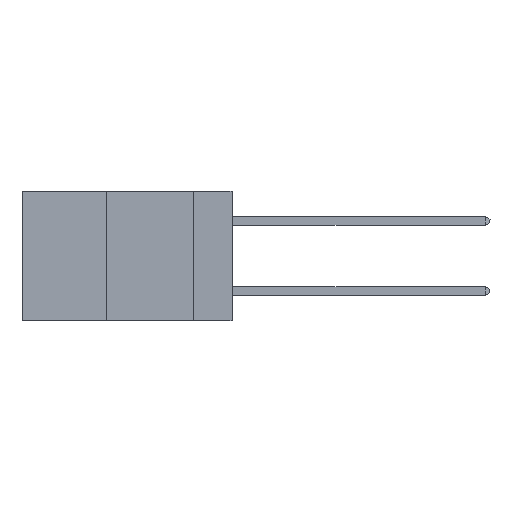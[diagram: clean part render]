
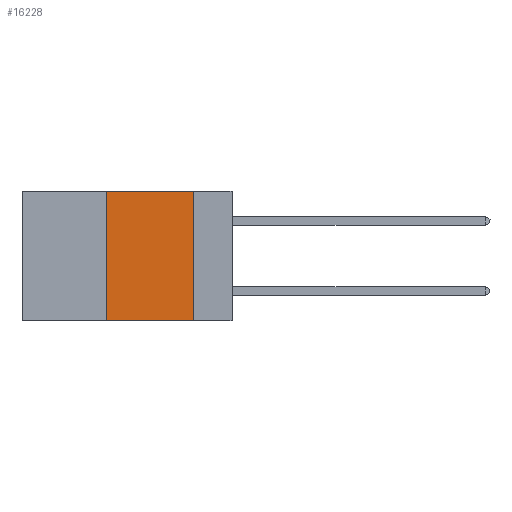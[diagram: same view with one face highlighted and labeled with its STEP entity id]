
A CAD part, left-side view. The second image highlights one B-rep face of the part: STEP entity #16228.
In plain terms, the highlighted planar face has unit normal (-1, 0, 0).
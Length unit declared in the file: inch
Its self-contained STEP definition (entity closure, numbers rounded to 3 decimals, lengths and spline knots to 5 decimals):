
#577 = EDGE_CURVE ( 'NONE', #12885, #24076, #1786, .T. ) ;
#1786 = LINE ( 'NONE', #29263, #32819 ) ;
#3264 = VECTOR ( 'NONE', #8563, 39.37008 ) ;
#3924 = CARTESIAN_POINT ( 'NONE',  ( 0., 0.36, -0.37 ) ) ;
#4252 = CARTESIAN_POINT ( 'NONE',  ( 0., 0.11, -0.37 ) ) ;
#4328 = CARTESIAN_POINT ( 'NONE',  ( 0., 0.36, 0. ) ) ;
#4683 = EDGE_CURVE ( 'NONE', #33873, #24076, #12021, .T. ) ;
#7788 = CARTESIAN_POINT ( 'NONE',  ( 0., 0.6, -0.37 ) ) ;
#8270 = FACE_OUTER_BOUND ( 'NONE', #40976, .T. ) ;
#8493 = LINE ( 'NONE', #4328, #3264 ) ;
#8563 = DIRECTION ( 'NONE',  ( 0., 0., 1. ) ) ;
#9419 = ORIENTED_EDGE ( 'NONE', *, *, #16579, .F. ) ;
#10001 = ORIENTED_EDGE ( 'NONE', *, *, #577, .F. ) ;
#10293 = DIRECTION ( 'NONE',  ( 0., 0., -1. ) ) ;
#12021 = LINE ( 'NONE', #7788, #29588 ) ;
#12531 = VERTEX_POINT ( 'NONE', #24932 ) ;
#12885 = VERTEX_POINT ( 'NONE', #38939 ) ;
#12928 = LINE ( 'NONE', #36656, #28137 ) ;
#16228 = ADVANCED_FACE ( 'NONE', ( #8270 ), #16256, .F. ) ;
#16256 = PLANE ( 'NONE',  #25536 ) ;
#16459 = ORIENTED_EDGE ( 'NONE', *, *, #4683, .T. ) ;
#16579 = EDGE_CURVE ( 'NONE', #12531, #12885, #12928, .T. ) ;
#18189 = DIRECTION ( 'NONE',  ( 0., -1., 0. ) ) ;
#19845 = DIRECTION ( 'NONE',  ( 1., 0., 0. ) ) ;
#24076 = VERTEX_POINT ( 'NONE', #4252 ) ;
#24932 = CARTESIAN_POINT ( 'NONE',  ( 0., 0.36, 0. ) ) ;
#25536 = AXIS2_PLACEMENT_3D ( 'NONE', #46469, #19845, #45824 ) ;
#26474 = ORIENTED_EDGE ( 'NONE', *, *, #32806, .F. ) ;
#26940 = DIRECTION ( 'NONE',  ( 0., -1., 0. ) ) ;
#28137 = VECTOR ( 'NONE', #18189, 39.37008 ) ;
#29263 = CARTESIAN_POINT ( 'NONE',  ( 0., 0.11, 0. ) ) ;
#29588 = VECTOR ( 'NONE', #26940, 39.37008 ) ;
#32806 = EDGE_CURVE ( 'NONE', #33873, #12531, #8493, .T. ) ;
#32819 = VECTOR ( 'NONE', #10293, 39.37008 ) ;
#33873 = VERTEX_POINT ( 'NONE', #3924 ) ;
#36656 = CARTESIAN_POINT ( 'NONE',  ( 0., 0.6, 0. ) ) ;
#38939 = CARTESIAN_POINT ( 'NONE',  ( 0., 0.11, 0. ) ) ;
#40976 = EDGE_LOOP ( 'NONE', ( #10001, #9419, #26474, #16459 ) ) ;
#45824 = DIRECTION ( 'NONE',  ( 0., 0., -1. ) ) ;
#46469 = CARTESIAN_POINT ( 'NONE',  ( 0., 0.6, 0. ) ) ;
